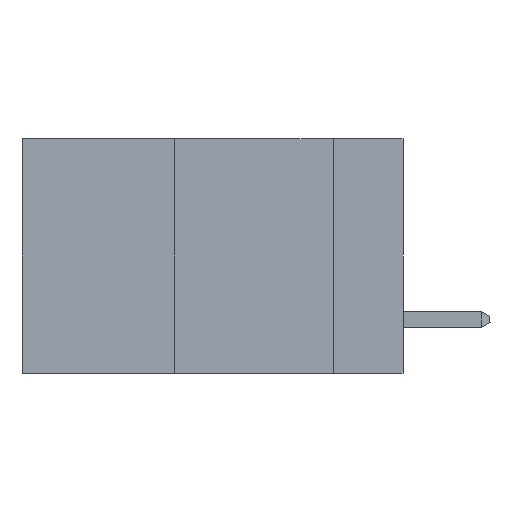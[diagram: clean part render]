
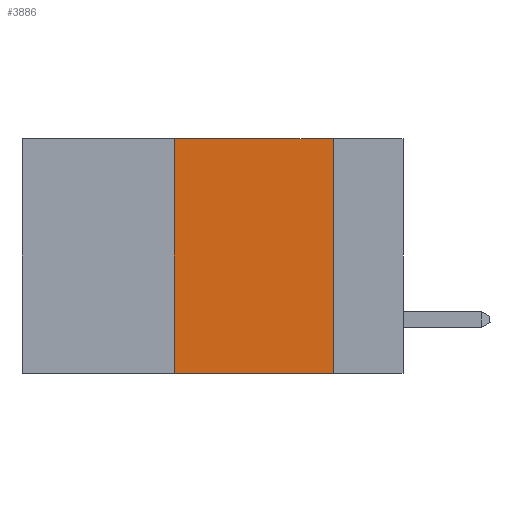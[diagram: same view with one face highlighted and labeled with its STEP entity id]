
A CAD part, left-side view. The second image highlights one B-rep face of the part: STEP entity #3886.
In plain terms, the highlighted planar face has unit normal (-1, 0, 0).
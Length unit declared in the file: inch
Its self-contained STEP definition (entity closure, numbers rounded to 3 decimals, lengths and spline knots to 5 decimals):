
#157 = CARTESIAN_POINT ( 'NONE',  ( 0., 0.36, 0. ) ) ;
#364 = DIRECTION ( 'NONE',  ( 0., 0., 1. ) ) ;
#2230 = CARTESIAN_POINT ( 'NONE',  ( 0., 0.11, -0.37 ) ) ;
#2450 = EDGE_CURVE ( 'NONE', #4511, #19035, #10453, .T. ) ;
#3232 = CARTESIAN_POINT ( 'NONE',  ( 0., 0.6, -0.37 ) ) ;
#3774 = PLANE ( 'NONE',  #5403 ) ;
#3886 = ADVANCED_FACE ( 'NONE', ( #4325 ), #3774, .F. ) ;
#4076 = CARTESIAN_POINT ( 'NONE',  ( 0., 0.36, 0. ) ) ;
#4325 = FACE_OUTER_BOUND ( 'NONE', #19664, .T. ) ;
#4511 = VERTEX_POINT ( 'NONE', #14276 ) ;
#5144 = LINE ( 'NONE', #157, #5639 ) ;
#5403 = AXIS2_PLACEMENT_3D ( 'NONE', #18335, #14859, #9211 ) ;
#5579 = EDGE_CURVE ( 'NONE', #17296, #19035, #8758, .T. ) ;
#5639 = VECTOR ( 'NONE', #364, 39.37008 ) ;
#6376 = VECTOR ( 'NONE', #8444, 39.37008 ) ;
#6486 = DIRECTION ( 'NONE',  ( 0., -1., 0. ) ) ;
#7050 = CARTESIAN_POINT ( 'NONE',  ( 0., 0.6, 0. ) ) ;
#8444 = DIRECTION ( 'NONE',  ( 0., -1., 0. ) ) ;
#8604 = EDGE_CURVE ( 'NONE', #17224, #4511, #18865, .T. ) ;
#8758 = LINE ( 'NONE', #3232, #13724 ) ;
#8846 = EDGE_CURVE ( 'NONE', #17296, #17224, #5144, .T. ) ;
#9211 = DIRECTION ( 'NONE',  ( 0., 0., -1. ) ) ;
#10215 = VECTOR ( 'NONE', #12252, 39.37008 ) ;
#10378 = ORIENTED_EDGE ( 'NONE', *, *, #2450, .F. ) ;
#10453 = LINE ( 'NONE', #15407, #10215 ) ;
#10838 = ORIENTED_EDGE ( 'NONE', *, *, #8604, .F. ) ;
#12252 = DIRECTION ( 'NONE',  ( 0., 0., -1. ) ) ;
#13724 = VECTOR ( 'NONE', #6486, 39.37008 ) ;
#13730 = ORIENTED_EDGE ( 'NONE', *, *, #5579, .T. ) ;
#14276 = CARTESIAN_POINT ( 'NONE',  ( 0., 0.11, 0. ) ) ;
#14859 = DIRECTION ( 'NONE',  ( 1., 0., 0. ) ) ;
#15407 = CARTESIAN_POINT ( 'NONE',  ( 0., 0.11, 0. ) ) ;
#16906 = ORIENTED_EDGE ( 'NONE', *, *, #8846, .F. ) ;
#17224 = VERTEX_POINT ( 'NONE', #4076 ) ;
#17296 = VERTEX_POINT ( 'NONE', #18443 ) ;
#18335 = CARTESIAN_POINT ( 'NONE',  ( 0., 0.6, 0. ) ) ;
#18443 = CARTESIAN_POINT ( 'NONE',  ( 0., 0.36, -0.37 ) ) ;
#18865 = LINE ( 'NONE', #7050, #6376 ) ;
#19035 = VERTEX_POINT ( 'NONE', #2230 ) ;
#19664 = EDGE_LOOP ( 'NONE', ( #10378, #10838, #16906, #13730 ) ) ;
